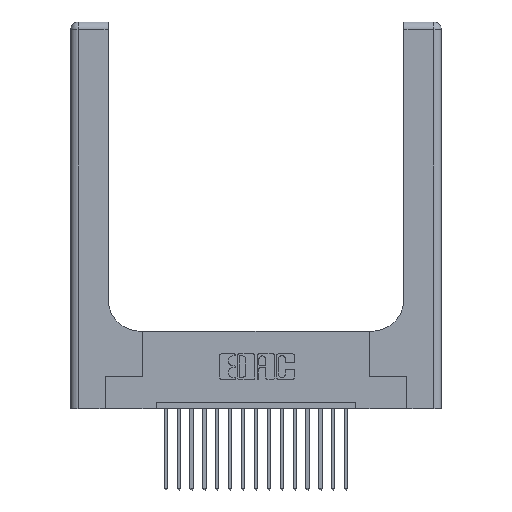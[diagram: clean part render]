
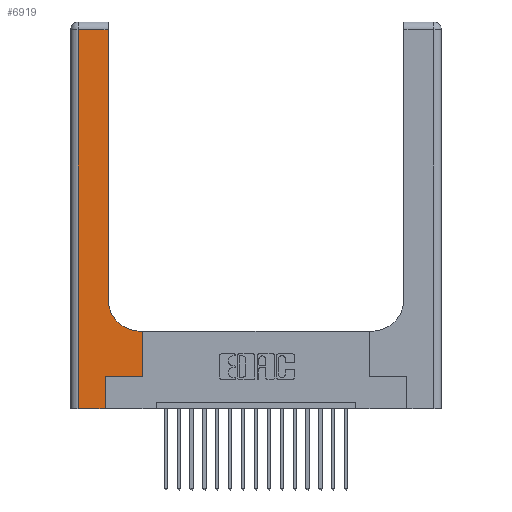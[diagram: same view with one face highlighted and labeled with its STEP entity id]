
A CAD part, top view. The second image highlights one B-rep face of the part: STEP entity #6919.
In plain terms, the highlighted planar face has unit normal (0, 0, 1).
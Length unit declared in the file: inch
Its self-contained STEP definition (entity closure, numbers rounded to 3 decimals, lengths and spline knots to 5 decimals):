
#372 = CARTESIAN_POINT ( 'NONE',  ( 0., 0., 0.37 ) ) ;
#422 = EDGE_CURVE ( 'NONE', #16160, #8277, #5030, .T. ) ;
#576 = CARTESIAN_POINT ( 'NONE',  ( 0.269, 0., 0.37 ) ) ;
#637 = EDGE_CURVE ( 'NONE', #18451, #3778, #10152, .T. ) ;
#743 = LINE ( 'NONE', #1800, #17502 ) ;
#831 = EDGE_CURVE ( 'NONE', #13716, #16160, #18865, .T. ) ;
#976 = DIRECTION ( 'NONE',  ( -1., 0., 0. ) ) ;
#1493 = CARTESIAN_POINT ( 'NONE',  ( 0.269, 0.25, 0.37 ) ) ;
#1642 = VECTOR ( 'NONE', #11039, 39.37008 ) ;
#1800 = CARTESIAN_POINT ( 'NONE',  ( 0.2915, 0.6, 0.37 ) ) ;
#1873 = VECTOR ( 'NONE', #2461, 39.37008 ) ;
#2072 = DIRECTION ( 'NONE',  ( 0., -1., 0. ) ) ;
#2121 = CARTESIAN_POINT ( 'NONE',  ( 0.06, 0., 0.37 ) ) ;
#2461 = DIRECTION ( 'NONE',  ( 0., 1., 0. ) ) ;
#2462 = VERTEX_POINT ( 'NONE', #2121 ) ;
#2551 = CARTESIAN_POINT ( 'NONE',  ( 0.5585, 0.6, 0.37 ) ) ;
#3064 = DIRECTION ( 'NONE',  ( 1., 0., 0. ) ) ;
#3279 = CIRCLE ( 'NONE', #15961, 0.25 ) ;
#3778 = VERTEX_POINT ( 'NONE', #2551 ) ;
#3807 = CARTESIAN_POINT ( 'NONE',  ( 0.5585, 0.25, 0.37 ) ) ;
#3915 = VECTOR ( 'NONE', #17484, 39.37008 ) ;
#4158 = CARTESIAN_POINT ( 'NONE',  ( 0.269, 0., 0.37 ) ) ;
#4236 = ORIENTED_EDGE ( 'NONE', *, *, #10228, .T. ) ;
#5030 = LINE ( 'NONE', #15576, #1642 ) ;
#5096 = VERTEX_POINT ( 'NONE', #10327 ) ;
#5954 = PLANE ( 'NONE',  #15963 ) ;
#5996 = CARTESIAN_POINT ( 'NONE',  ( 0.5415, 0.85, 0.37 ) ) ;
#6135 = DIRECTION ( 'NONE',  ( 1., 0., 0. ) ) ;
#6919 = ADVANCED_FACE ( 'NONE', ( #11767 ), #5954, .F. ) ;
#7120 = CARTESIAN_POINT ( 'NONE',  ( 0.5585, 0.25, 0.37 ) ) ;
#7443 = EDGE_CURVE ( 'NONE', #12768, #15854, #11260, .T. ) ;
#7485 = DIRECTION ( 'NONE',  ( 0., 1., 0. ) ) ;
#7739 = VECTOR ( 'NONE', #7485, 39.37008 ) ;
#8262 = ORIENTED_EDGE ( 'NONE', *, *, #7443, .T. ) ;
#8277 = VERTEX_POINT ( 'NONE', #15272 ) ;
#8492 = EDGE_CURVE ( 'NONE', #3778, #5096, #743, .T. ) ;
#8639 = CARTESIAN_POINT ( 'NONE',  ( 0.2915, 3., 0.37 ) ) ;
#9071 = DIRECTION ( 'NONE',  ( 0., 0., -1. ) ) ;
#9196 = ORIENTED_EDGE ( 'NONE', *, *, #831, .T. ) ;
#9404 = ORIENTED_EDGE ( 'NONE', *, *, #422, .T. ) ;
#10061 = CARTESIAN_POINT ( 'NONE',  ( 0.2915, 2.94, 0.37 ) ) ;
#10152 = LINE ( 'NONE', #7120, #1873 ) ;
#10228 = EDGE_CURVE ( 'NONE', #8277, #2462, #18178, .T. ) ;
#10327 = CARTESIAN_POINT ( 'NONE',  ( 0.5415, 0.6, 0.37 ) ) ;
#10508 = LINE ( 'NONE', #372, #3915 ) ;
#10912 = CARTESIAN_POINT ( 'NONE',  ( 0.269, 0.25, 0.37 ) ) ;
#11039 = DIRECTION ( 'NONE',  ( -1., 0., 0. ) ) ;
#11260 = LINE ( 'NONE', #4158, #19978 ) ;
#11437 = ORIENTED_EDGE ( 'NONE', *, *, #19525, .T. ) ;
#11767 = FACE_OUTER_BOUND ( 'NONE', #19069, .T. ) ;
#12768 = VERTEX_POINT ( 'NONE', #576 ) ;
#12823 = DIRECTION ( 'NONE',  ( -1., 0., 0. ) ) ;
#12875 = ORIENTED_EDGE ( 'NONE', *, *, #637, .T. ) ;
#13644 = ORIENTED_EDGE ( 'NONE', *, *, #13685, .T. ) ;
#13679 = EDGE_CURVE ( 'NONE', #15854, #18451, #14682, .T. ) ;
#13685 = EDGE_CURVE ( 'NONE', #5096, #13716, #3279, .T. ) ;
#13716 = VERTEX_POINT ( 'NONE', #16917 ) ;
#13733 = VECTOR ( 'NONE', #3064, 39.37008 ) ;
#14074 = VECTOR ( 'NONE', #2072, 39.37008 ) ;
#14682 = LINE ( 'NONE', #1493, #13733 ) ;
#14735 = DIRECTION ( 'NONE',  ( 0., 1., 0. ) ) ;
#15117 = DIRECTION ( 'NONE',  ( 0., 0., -1. ) ) ;
#15272 = CARTESIAN_POINT ( 'NONE',  ( 0.06, 2.94, 0.37 ) ) ;
#15576 = CARTESIAN_POINT ( 'NONE',  ( 0., 2.94, 0.37 ) ) ;
#15854 = VERTEX_POINT ( 'NONE', #10912 ) ;
#15961 = AXIS2_PLACEMENT_3D ( 'NONE', #5996, #9071, #6135 ) ;
#15963 = AXIS2_PLACEMENT_3D ( 'NONE', #18021, #15117, #976 ) ;
#16160 = VERTEX_POINT ( 'NONE', #10061 ) ;
#16192 = ORIENTED_EDGE ( 'NONE', *, *, #13679, .T. ) ;
#16917 = CARTESIAN_POINT ( 'NONE',  ( 0.2915, 0.85, 0.37 ) ) ;
#17484 = DIRECTION ( 'NONE',  ( 1., 0., 0. ) ) ;
#17502 = VECTOR ( 'NONE', #12823, 39.37008 ) ;
#18021 = CARTESIAN_POINT ( 'NONE',  ( 0., 3., 0.37 ) ) ;
#18043 = ORIENTED_EDGE ( 'NONE', *, *, #8492, .T. ) ;
#18178 = LINE ( 'NONE', #19331, #14074 ) ;
#18451 = VERTEX_POINT ( 'NONE', #3807 ) ;
#18865 = LINE ( 'NONE', #8639, #7739 ) ;
#19069 = EDGE_LOOP ( 'NONE', ( #9196, #9404, #4236, #11437, #8262, #16192, #12875, #18043, #13644 ) ) ;
#19331 = CARTESIAN_POINT ( 'NONE',  ( 0.06, 3., 0.37 ) ) ;
#19525 = EDGE_CURVE ( 'NONE', #2462, #12768, #10508, .T. ) ;
#19978 = VECTOR ( 'NONE', #14735, 39.37008 ) ;
